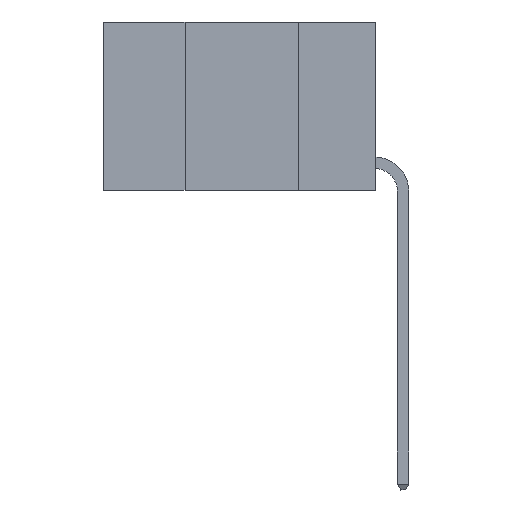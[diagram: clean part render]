
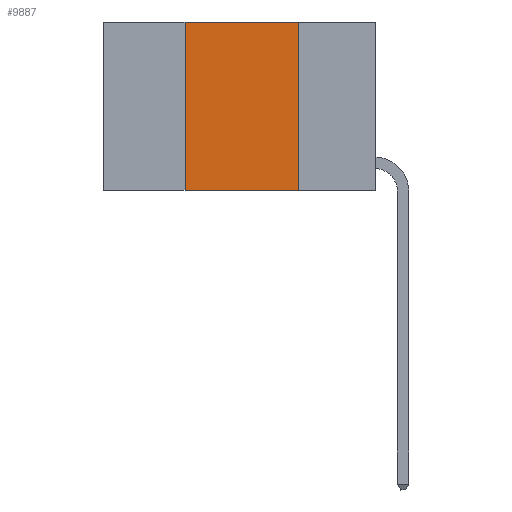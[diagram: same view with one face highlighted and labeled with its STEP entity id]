
A CAD part, left-side view. The second image highlights one B-rep face of the part: STEP entity #9887.
In plain terms, the highlighted planar face has unit normal (-1, 0, 0).
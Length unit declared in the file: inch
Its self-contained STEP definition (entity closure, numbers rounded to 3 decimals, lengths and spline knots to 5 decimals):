
#719 = EDGE_CURVE ( 'NONE', #15645, #8752, #4193, .T. ) ;
#813 = CARTESIAN_POINT ( 'NONE',  ( 0., 0.42, 0. ) ) ;
#928 = LINE ( 'NONE', #12516, #9272 ) ;
#2805 = EDGE_CURVE ( 'NONE', #8752, #13089, #5629, .T. ) ;
#3053 = PLANE ( 'NONE',  #14652 ) ;
#3439 = DIRECTION ( 'NONE',  ( 0., 0., -1. ) ) ;
#3527 = EDGE_CURVE ( 'NONE', #13089, #10524, #8477, .T. ) ;
#3804 = DIRECTION ( 'NONE',  ( 0., -1., 0. ) ) ;
#4193 = LINE ( 'NONE', #14223, #10002 ) ;
#4197 = FACE_OUTER_BOUND ( 'NONE', #8451, .T. ) ;
#4628 = CARTESIAN_POINT ( 'NONE',  ( 0., 0.17, 0. ) ) ;
#5629 = LINE ( 'NONE', #15807, #10574 ) ;
#6432 = CARTESIAN_POINT ( 'NONE',  ( 0., 0.6, 0. ) ) ;
#6508 = DIRECTION ( 'NONE',  ( 0., 0., -1. ) ) ;
#6583 = DIRECTION ( 'NONE',  ( 0., 0., 1. ) ) ;
#7339 = ORIENTED_EDGE ( 'NONE', *, *, #11015, .T. ) ;
#8053 = ORIENTED_EDGE ( 'NONE', *, *, #719, .F. ) ;
#8241 = ORIENTED_EDGE ( 'NONE', *, *, #2805, .F. ) ;
#8451 = EDGE_LOOP ( 'NONE', ( #8707, #8241, #8053, #7339 ) ) ;
#8477 = LINE ( 'NONE', #14856, #15688 ) ;
#8707 = ORIENTED_EDGE ( 'NONE', *, *, #3527, .F. ) ;
#8752 = VERTEX_POINT ( 'NONE', #813 ) ;
#9272 = VECTOR ( 'NONE', #13608, 39.37008 ) ;
#9887 = ADVANCED_FACE ( 'NONE', ( #4197 ), #3053, .F. ) ;
#10002 = VECTOR ( 'NONE', #6583, 39.37008 ) ;
#10524 = VERTEX_POINT ( 'NONE', #10565 ) ;
#10565 = CARTESIAN_POINT ( 'NONE',  ( 0., 0.17, -0.37 ) ) ;
#10574 = VECTOR ( 'NONE', #3804, 39.37008 ) ;
#11015 = EDGE_CURVE ( 'NONE', #15645, #10524, #928, .T. ) ;
#12516 = CARTESIAN_POINT ( 'NONE',  ( 0., 0.6, -0.37 ) ) ;
#12963 = DIRECTION ( 'NONE',  ( 1., 0., 0. ) ) ;
#13089 = VERTEX_POINT ( 'NONE', #4628 ) ;
#13608 = DIRECTION ( 'NONE',  ( 0., -1., 0. ) ) ;
#14223 = CARTESIAN_POINT ( 'NONE',  ( 0., 0.42, 0. ) ) ;
#14652 = AXIS2_PLACEMENT_3D ( 'NONE', #6432, #12963, #6508 ) ;
#14856 = CARTESIAN_POINT ( 'NONE',  ( 0., 0.17, 0. ) ) ;
#15636 = CARTESIAN_POINT ( 'NONE',  ( 0., 0.42, -0.37 ) ) ;
#15645 = VERTEX_POINT ( 'NONE', #15636 ) ;
#15688 = VECTOR ( 'NONE', #3439, 39.37008 ) ;
#15807 = CARTESIAN_POINT ( 'NONE',  ( 0., 0.6, 0. ) ) ;
